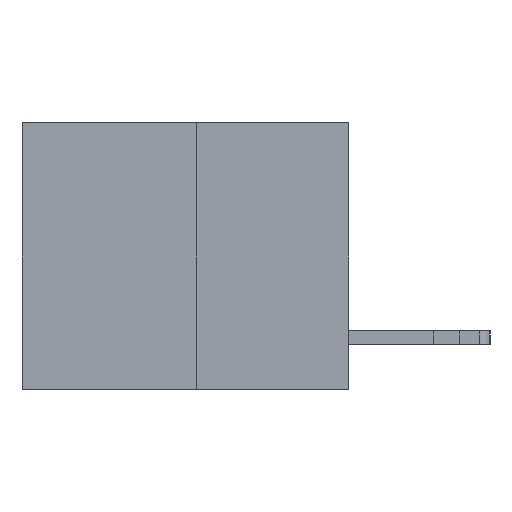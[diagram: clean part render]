
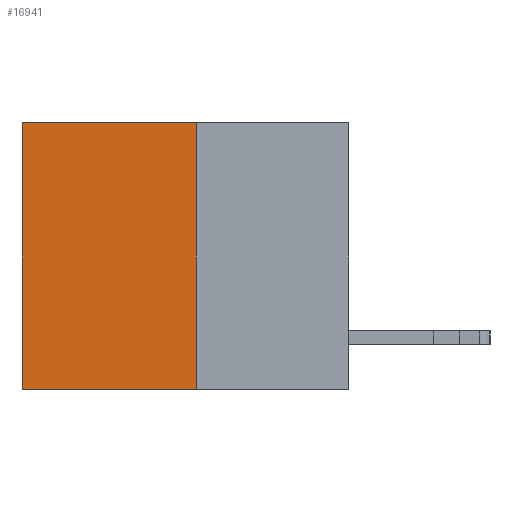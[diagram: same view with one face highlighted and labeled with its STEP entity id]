
A CAD part, left-side view. The second image highlights one B-rep face of the part: STEP entity #16941.
In plain terms, the highlighted planar face has unit normal (-1, 0, 0).
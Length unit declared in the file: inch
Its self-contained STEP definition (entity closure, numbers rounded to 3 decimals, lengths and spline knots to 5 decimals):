
#413 = AXIS2_PLACEMENT_3D ( 'NONE', #10443, #11894, #5039 ) ;
#1992 = CARTESIAN_POINT ( 'NONE',  ( 0.3165, 0.28, -0.49 ) ) ;
#2684 = VECTOR ( 'NONE', #12885, 39.37008 ) ;
#4094 = LINE ( 'NONE', #1992, #5181 ) ;
#4331 = CARTESIAN_POINT ( 'NONE',  ( 0.3165, 0.28, -0.49 ) ) ;
#4461 = CARTESIAN_POINT ( 'NONE',  ( 0.3165, 0.28, 0. ) ) ;
#4552 = DIRECTION ( 'NONE',  ( 0., 1., 0. ) ) ;
#5039 = DIRECTION ( 'NONE',  ( 0., 0., -1. ) ) ;
#5181 = VECTOR ( 'NONE', #8818, 39.37008 ) ;
#6089 = CARTESIAN_POINT ( 'NONE',  ( 0.3165, 0.28, 0. ) ) ;
#6605 = EDGE_CURVE ( 'NONE', #10776, #21921, #9451, .T. ) ;
#6923 = PLANE ( 'NONE',  #413 ) ;
#7313 = CARTESIAN_POINT ( 'NONE',  ( 0.3165, 0.28, -0.49 ) ) ;
#7524 = CARTESIAN_POINT ( 'NONE',  ( 0.3165, 0.6, -0.49 ) ) ;
#7577 = VECTOR ( 'NONE', #4552, 39.37008 ) ;
#8818 = DIRECTION ( 'NONE',  ( 0., 1., 0. ) ) ;
#9193 = VECTOR ( 'NONE', #19256, 39.37008 ) ;
#9451 = LINE ( 'NONE', #4461, #7577 ) ;
#10443 = CARTESIAN_POINT ( 'NONE',  ( 0.3165, 0.28, -0.49 ) ) ;
#10776 = VERTEX_POINT ( 'NONE', #6089 ) ;
#11242 = EDGE_LOOP ( 'NONE', ( #14721, #11586, #11829, #21869 ) ) ;
#11586 = ORIENTED_EDGE ( 'NONE', *, *, #19185, .F. ) ;
#11829 = ORIENTED_EDGE ( 'NONE', *, *, #12166, .F. ) ;
#11894 = DIRECTION ( 'NONE',  ( 1., 0., 0. ) ) ;
#12166 = EDGE_CURVE ( 'NONE', #10776, #20672, #16681, .T. ) ;
#12885 = DIRECTION ( 'NONE',  ( 0., 0., -1. ) ) ;
#14025 = LINE ( 'NONE', #19117, #9193 ) ;
#14160 = CARTESIAN_POINT ( 'NONE',  ( 0.3165, 0.6, 0. ) ) ;
#14721 = ORIENTED_EDGE ( 'NONE', *, *, #20577, .T. ) ;
#16681 = LINE ( 'NONE', #4331, #2684 ) ;
#16941 = ADVANCED_FACE ( 'NONE', ( #19277 ), #6923, .F. ) ;
#19117 = CARTESIAN_POINT ( 'NONE',  ( 0.3165, 0.6, -0.49 ) ) ;
#19185 = EDGE_CURVE ( 'NONE', #20672, #20792, #4094, .T. ) ;
#19256 = DIRECTION ( 'NONE',  ( 0., 0., -1. ) ) ;
#19277 = FACE_OUTER_BOUND ( 'NONE', #11242, .T. ) ;
#20577 = EDGE_CURVE ( 'NONE', #21921, #20792, #14025, .T. ) ;
#20672 = VERTEX_POINT ( 'NONE', #7313 ) ;
#20792 = VERTEX_POINT ( 'NONE', #7524 ) ;
#21869 = ORIENTED_EDGE ( 'NONE', *, *, #6605, .T. ) ;
#21921 = VERTEX_POINT ( 'NONE', #14160 ) ;
